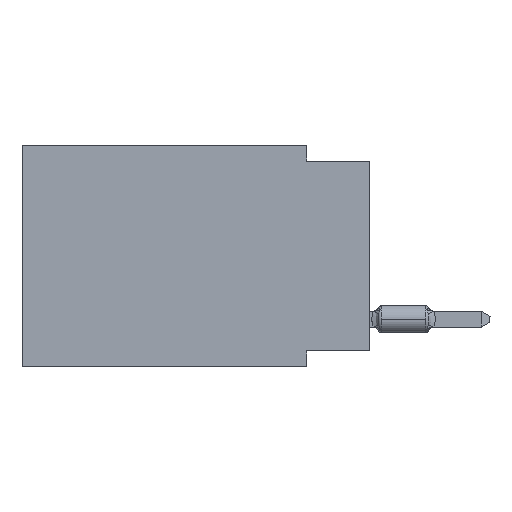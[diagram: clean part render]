
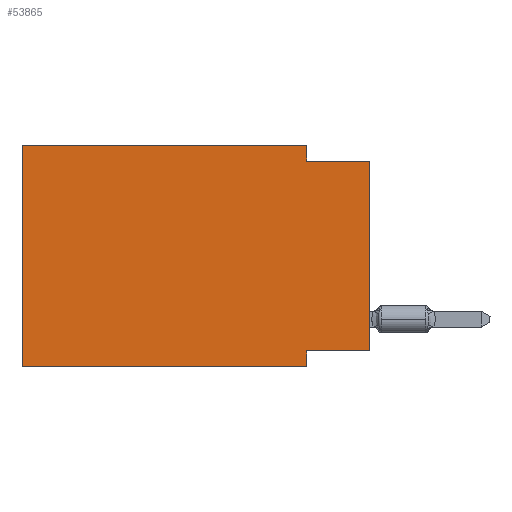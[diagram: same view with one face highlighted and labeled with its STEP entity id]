
A CAD part, left-side view. The second image highlights one B-rep face of the part: STEP entity #53865.
In plain terms, the highlighted planar face has unit normal (-1, 0, 0).
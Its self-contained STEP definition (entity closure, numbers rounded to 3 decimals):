
#739 = DIRECTION ( 'NONE',  ( 0., 0., -1. ) ) ;
#3640 = EDGE_CURVE ( 'NONE', #72493, #87794, #92990, .T. ) ;
#4861 = LINE ( 'NONE', #82036, #52909 ) ;
#5272 = DIRECTION ( 'NONE',  ( 0., 0., 1. ) ) ;
#5531 = CARTESIAN_POINT ( 'NONE',  ( 0., 2.54, 0. ) ) ;
#7344 = VERTEX_POINT ( 'NONE', #33540 ) ;
#12959 = LINE ( 'NONE', #44136, #21667 ) ;
#18225 = LINE ( 'NONE', #49398, #26277 ) ;
#18644 = VERTEX_POINT ( 'NONE', #26229 ) ;
#20135 = EDGE_CURVE ( 'NONE', #18644, #7344, #95815, .T. ) ;
#21470 = EDGE_CURVE ( 'NONE', #98092, #51040, #12959, .T. ) ;
#21667 = VECTOR ( 'NONE', #5272, 1000. ) ;
#23440 = CARTESIAN_POINT ( 'NONE',  ( 0., 2.54, 0. ) ) ;
#24061 = DIRECTION ( 'NONE',  ( 0., 0., -1. ) ) ;
#24761 = CARTESIAN_POINT ( 'NONE',  ( 0., 2.54, -8.89 ) ) ;
#25457 = VECTOR ( 'NONE', #63402, 1000. ) ;
#25569 = PLANE ( 'NONE',  #37189 ) ;
#26229 = CARTESIAN_POINT ( 'NONE',  ( 0., 2.54, -8.255 ) ) ;
#26277 = VECTOR ( 'NONE', #80591, 1000. ) ;
#27167 = ORIENTED_EDGE ( 'NONE', *, *, #20135, .F. ) ;
#27604 = VECTOR ( 'NONE', #73836, 1000. ) ;
#28972 = CARTESIAN_POINT ( 'NONE',  ( 0., 13.97, 0. ) ) ;
#30920 = CARTESIAN_POINT ( 'NONE',  ( 0., 13.97, -8.89 ) ) ;
#31209 = CARTESIAN_POINT ( 'NONE',  ( 0., 13.97, 0. ) ) ;
#33540 = CARTESIAN_POINT ( 'NONE',  ( 0., 2.54, -8.89 ) ) ;
#37189 = AXIS2_PLACEMENT_3D ( 'NONE', #95607, #39880, #24061 ) ;
#39880 = DIRECTION ( 'NONE',  ( 1., 0., 0. ) ) ;
#41278 = CARTESIAN_POINT ( 'NONE',  ( 0., 0., -8.255 ) ) ;
#42168 = CARTESIAN_POINT ( 'NONE',  ( 0., 0., -0.635 ) ) ;
#43191 = DIRECTION ( 'NONE',  ( 0., 1., 0. ) ) ;
#44136 = CARTESIAN_POINT ( 'NONE',  ( 0., 13.97, 0. ) ) ;
#46223 = ORIENTED_EDGE ( 'NONE', *, *, #74540, .F. ) ;
#46808 = ORIENTED_EDGE ( 'NONE', *, *, #61442, .T. ) ;
#47325 = ORIENTED_EDGE ( 'NONE', *, *, #3640, .F. ) ;
#49398 = CARTESIAN_POINT ( 'NONE',  ( 0., 0., 0. ) ) ;
#51040 = VERTEX_POINT ( 'NONE', #28972 ) ;
#51576 = VERTEX_POINT ( 'NONE', #41278 ) ;
#52909 = VECTOR ( 'NONE', #43191, 1000. ) ;
#53865 = ADVANCED_FACE ( 'NONE', ( #94096 ), #25569, .F. ) ;
#60759 = DIRECTION ( 'NONE',  ( 0., 0., -1. ) ) ;
#61442 = EDGE_CURVE ( 'NONE', #51576, #68011, #18225, .T. ) ;
#62084 = ORIENTED_EDGE ( 'NONE', *, *, #92781, .T. ) ;
#63402 = DIRECTION ( 'NONE',  ( 0., -1., 0. ) ) ;
#63443 = CARTESIAN_POINT ( 'NONE',  ( 0., 13.97, -8.89 ) ) ;
#66100 = CARTESIAN_POINT ( 'NONE',  ( 0., 0., -0.635 ) ) ;
#66162 = LINE ( 'NONE', #42168, #27604 ) ;
#68011 = VERTEX_POINT ( 'NONE', #66100 ) ;
#72338 = VECTOR ( 'NONE', #739, 1000. ) ;
#72493 = VERTEX_POINT ( 'NONE', #5531 ) ;
#73836 = DIRECTION ( 'NONE',  ( 0., -1., 0. ) ) ;
#74540 = EDGE_CURVE ( 'NONE', #87794, #68011, #66162, .T. ) ;
#75895 = DIRECTION ( 'NONE',  ( 0., -1., 0. ) ) ;
#78032 = ORIENTED_EDGE ( 'NONE', *, *, #88119, .F. ) ;
#78226 = LINE ( 'NONE', #31209, #25457 ) ;
#78602 = EDGE_LOOP ( 'NONE', ( #46808, #46223, #47325, #78032, #83507, #62084, #27167, #93223 ) ) ;
#80591 = DIRECTION ( 'NONE',  ( 0., 0., 1. ) ) ;
#82036 = CARTESIAN_POINT ( 'NONE',  ( 0., 0., -8.255 ) ) ;
#82828 = VECTOR ( 'NONE', #75895, 1000. ) ;
#83361 = VECTOR ( 'NONE', #60759, 1000. ) ;
#83507 = ORIENTED_EDGE ( 'NONE', *, *, #21470, .F. ) ;
#87794 = VERTEX_POINT ( 'NONE', #89047 ) ;
#88119 = EDGE_CURVE ( 'NONE', #51040, #72493, #78226, .T. ) ;
#89047 = CARTESIAN_POINT ( 'NONE',  ( 0., 2.54, -0.635 ) ) ;
#92780 = LINE ( 'NONE', #30920, #82828 ) ;
#92781 = EDGE_CURVE ( 'NONE', #98092, #7344, #92780, .T. ) ;
#92990 = LINE ( 'NONE', #23440, #83361 ) ;
#93223 = ORIENTED_EDGE ( 'NONE', *, *, #99114, .F. ) ;
#94096 = FACE_OUTER_BOUND ( 'NONE', #78602, .T. ) ;
#95607 = CARTESIAN_POINT ( 'NONE',  ( 0., 13.97, 0. ) ) ;
#95815 = LINE ( 'NONE', #24761, #72338 ) ;
#98092 = VERTEX_POINT ( 'NONE', #63443 ) ;
#99114 = EDGE_CURVE ( 'NONE', #51576, #18644, #4861, .T. ) ;
